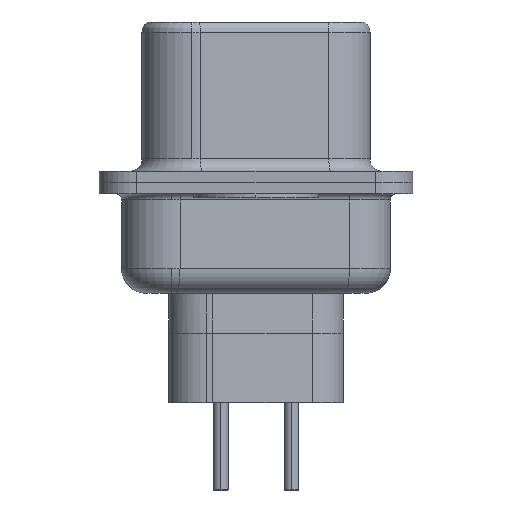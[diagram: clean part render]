
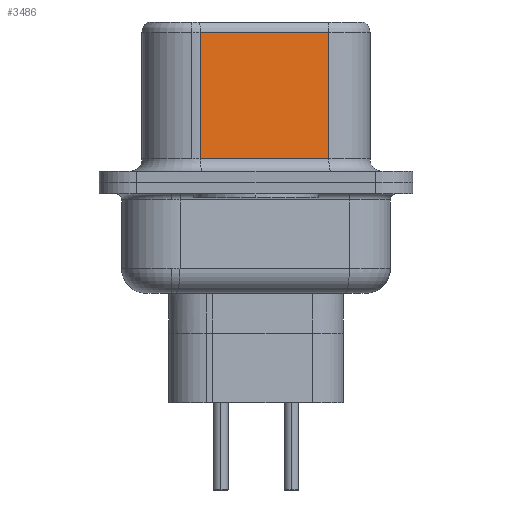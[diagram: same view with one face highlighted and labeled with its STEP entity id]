
A CAD part, left-side view. The second image highlights one B-rep face of the part: STEP entity #3486.
In plain terms, the highlighted planar face has unit normal (-0.985, -0.174, 0).
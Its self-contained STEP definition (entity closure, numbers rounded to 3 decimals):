
#139 = CARTESIAN_POINT ( 'NONE',  ( 3.665, 2.233, 6.52 ) ) ;
#1008 = DIRECTION ( 'NONE',  ( 0., 0., -1. ) ) ;
#1129 = DIRECTION ( 'NONE',  ( -0.174, 0.985, 0. ) ) ;
#1935 = ORIENTED_EDGE ( 'NONE', *, *, #14843, .F. ) ;
#2251 = CARTESIAN_POINT ( 'NONE',  ( 4.575, -2.927, 0.95 ) ) ;
#2438 = DIRECTION ( 'NONE',  ( 0.174, -0.985, 0. ) ) ;
#3232 = EDGE_LOOP ( 'NONE', ( #1935, #9302, #14973, #8743 ) ) ;
#3486 = ADVANCED_FACE ( 'NONE', ( #12848 ), #15543, .F. ) ;
#4463 = EDGE_CURVE ( 'NONE', #11396, #16081, #14598, .T. ) ;
#4760 = DIRECTION ( 'NONE',  ( -0.174, 0.985, 0. ) ) ;
#4841 = CARTESIAN_POINT ( 'NONE',  ( 4.575, -2.927, 6.52 ) ) ;
#4919 = LINE ( 'NONE', #5097, #6926 ) ;
#5097 = CARTESIAN_POINT ( 'NONE',  ( 4.575, -2.927, 6.02 ) ) ;
#5909 = CARTESIAN_POINT ( 'NONE',  ( 3.665, 2.233, 0.95 ) ) ;
#6328 = AXIS2_PLACEMENT_3D ( 'NONE', #4841, #13203, #4760 ) ;
#6553 = CARTESIAN_POINT ( 'NONE',  ( 3.665, 2.233, 6.02 ) ) ;
#6661 = VECTOR ( 'NONE', #1008, 1000. ) ;
#6803 = EDGE_CURVE ( 'NONE', #12279, #11396, #15072, .T. ) ;
#6926 = VECTOR ( 'NONE', #1129, 1000. ) ;
#7844 = CARTESIAN_POINT ( 'NONE',  ( 4.575, -2.927, 6.52 ) ) ;
#8395 = VECTOR ( 'NONE', #15159, 1000. ) ;
#8743 = ORIENTED_EDGE ( 'NONE', *, *, #4463, .T. ) ;
#9302 = ORIENTED_EDGE ( 'NONE', *, *, #14412, .T. ) ;
#10408 = CARTESIAN_POINT ( 'NONE',  ( 4.575, -2.927, 6.02 ) ) ;
#11396 = VERTEX_POINT ( 'NONE', #5909 ) ;
#11754 = VECTOR ( 'NONE', #2438, 1000. ) ;
#12279 = VERTEX_POINT ( 'NONE', #6553 ) ;
#12848 = FACE_OUTER_BOUND ( 'NONE', #3232, .T. ) ;
#13100 = CARTESIAN_POINT ( 'NONE',  ( 4.575, -2.927, 0.95 ) ) ;
#13203 = DIRECTION ( 'NONE',  ( 0.985, 0.174, 0. ) ) ;
#14412 = EDGE_CURVE ( 'NONE', #14447, #12279, #4919, .T. ) ;
#14447 = VERTEX_POINT ( 'NONE', #10408 ) ;
#14598 = LINE ( 'NONE', #2251, #11754 ) ;
#14843 = EDGE_CURVE ( 'NONE', #14447, #16081, #14871, .T. ) ;
#14871 = LINE ( 'NONE', #7844, #6661 ) ;
#14973 = ORIENTED_EDGE ( 'NONE', *, *, #6803, .T. ) ;
#15072 = LINE ( 'NONE', #139, #8395 ) ;
#15159 = DIRECTION ( 'NONE',  ( 0., 0., -1. ) ) ;
#15543 = PLANE ( 'NONE',  #6328 ) ;
#16081 = VERTEX_POINT ( 'NONE', #13100 ) ;
